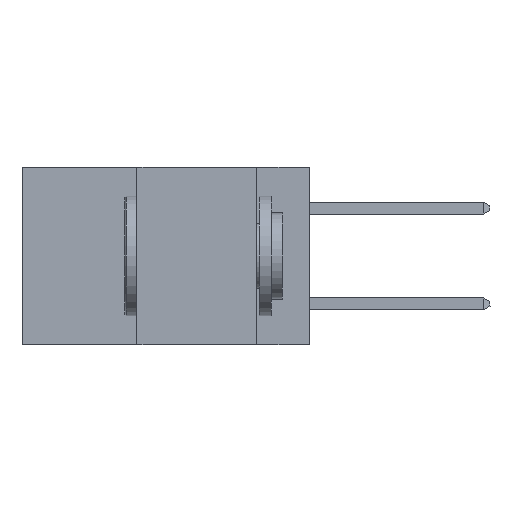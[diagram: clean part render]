
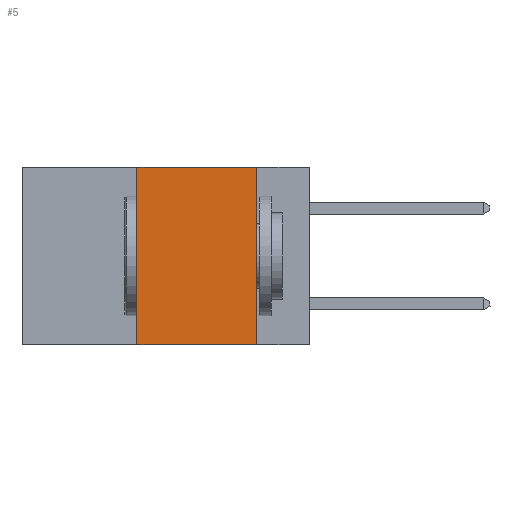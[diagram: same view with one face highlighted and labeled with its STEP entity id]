
A CAD part, left-side view. The second image highlights one B-rep face of the part: STEP entity #5.
In plain terms, the highlighted planar face has unit normal (-1, 0, 0).
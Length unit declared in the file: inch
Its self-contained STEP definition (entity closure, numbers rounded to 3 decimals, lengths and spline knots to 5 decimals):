
#5 = ADVANCED_FACE ( 'NONE', ( #6361 ), #5806, .F. ) ;
#74 = VECTOR ( 'NONE', #3827, 39.37008 ) ;
#329 = DIRECTION ( 'NONE',  ( 0., -1., 0. ) ) ;
#514 = LINE ( 'NONE', #1843, #10843 ) ;
#712 = LINE ( 'NONE', #8511, #11039 ) ;
#1329 = EDGE_LOOP ( 'NONE', ( #11177, #5133, #8674, #10163 ) ) ;
#1430 = DIRECTION ( 'NONE',  ( 0., 0., -1. ) ) ;
#1797 = DIRECTION ( 'NONE',  ( 0., -1., 0. ) ) ;
#1843 = CARTESIAN_POINT ( 'NONE',  ( 0., 0.6, -0.37 ) ) ;
#1944 = CARTESIAN_POINT ( 'NONE',  ( 0., 0.36, 0. ) ) ;
#2208 = CARTESIAN_POINT ( 'NONE',  ( 0., 0.6, 0. ) ) ;
#2575 = DIRECTION ( 'NONE',  ( 0., 0., -1. ) ) ;
#3827 = DIRECTION ( 'NONE',  ( 0., 0., 1. ) ) ;
#3946 = VERTEX_POINT ( 'NONE', #10099 ) ;
#4100 = LINE ( 'NONE', #5501, #6869 ) ;
#4518 = CARTESIAN_POINT ( 'NONE',  ( 0., 0.11, -0.37 ) ) ;
#5061 = AXIS2_PLACEMENT_3D ( 'NONE', #2208, #7175, #1430 ) ;
#5133 = ORIENTED_EDGE ( 'NONE', *, *, #7793, .F. ) ;
#5363 = LINE ( 'NONE', #1944, #74 ) ;
#5501 = CARTESIAN_POINT ( 'NONE',  ( 0., 0.6, 0. ) ) ;
#5806 = PLANE ( 'NONE',  #5061 ) ;
#5861 = EDGE_CURVE ( 'NONE', #12843, #3946, #5363, .T. ) ;
#5972 = VERTEX_POINT ( 'NONE', #4518 ) ;
#6361 = FACE_OUTER_BOUND ( 'NONE', #1329, .T. ) ;
#6599 = CARTESIAN_POINT ( 'NONE',  ( 0., 0.11, 0. ) ) ;
#6869 = VECTOR ( 'NONE', #329, 39.37008 ) ;
#7175 = DIRECTION ( 'NONE',  ( 1., 0., 0. ) ) ;
#7185 = EDGE_CURVE ( 'NONE', #11231, #5972, #712, .T. ) ;
#7793 = EDGE_CURVE ( 'NONE', #3946, #11231, #4100, .T. ) ;
#8511 = CARTESIAN_POINT ( 'NONE',  ( 0., 0.11, 0. ) ) ;
#8674 = ORIENTED_EDGE ( 'NONE', *, *, #5861, .F. ) ;
#10099 = CARTESIAN_POINT ( 'NONE',  ( 0., 0.36, 0. ) ) ;
#10163 = ORIENTED_EDGE ( 'NONE', *, *, #12171, .T. ) ;
#10843 = VECTOR ( 'NONE', #1797, 39.37008 ) ;
#10884 = CARTESIAN_POINT ( 'NONE',  ( 0., 0.36, -0.37 ) ) ;
#11039 = VECTOR ( 'NONE', #2575, 39.37008 ) ;
#11177 = ORIENTED_EDGE ( 'NONE', *, *, #7185, .F. ) ;
#11231 = VERTEX_POINT ( 'NONE', #6599 ) ;
#12171 = EDGE_CURVE ( 'NONE', #12843, #5972, #514, .T. ) ;
#12843 = VERTEX_POINT ( 'NONE', #10884 ) ;
